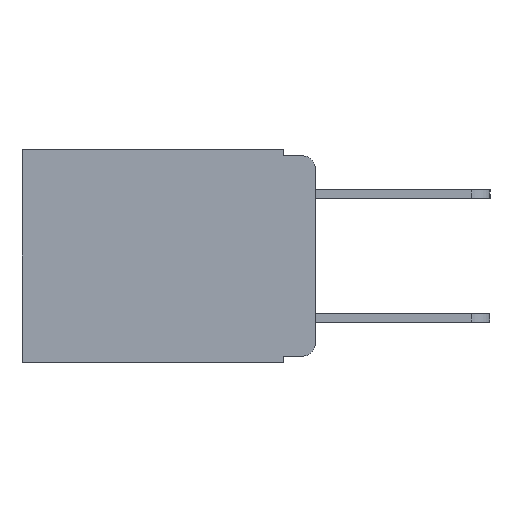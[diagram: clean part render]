
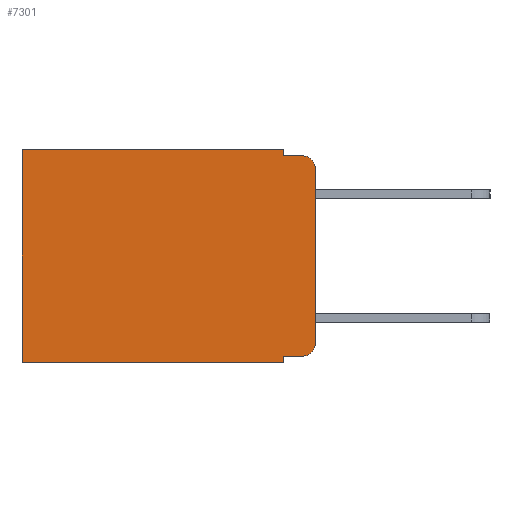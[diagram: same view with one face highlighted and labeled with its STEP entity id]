
A CAD part, left-side view. The second image highlights one B-rep face of the part: STEP entity #7301.
In plain terms, the highlighted planar face has unit normal (-1, 0, 0).
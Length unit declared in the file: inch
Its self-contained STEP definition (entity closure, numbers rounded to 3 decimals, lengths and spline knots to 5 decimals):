
#232 = DIRECTION ( 'NONE',  ( 0., 0., -1. ) ) ;
#924 = LINE ( 'NONE', #11847, #10627 ) ;
#1028 = VECTOR ( 'NONE', #232, 39.37008 ) ;
#1102 = DIRECTION ( 'NONE',  ( 0., 0., -1. ) ) ;
#1113 = DIRECTION ( 'NONE',  ( -1., 0., 0. ) ) ;
#1118 = AXIS2_PLACEMENT_3D ( 'NONE', #11183, #9287, #4000 ) ;
#1119 = CARTESIAN_POINT ( 'NONE',  ( 0.298, 0.02, -0.313 ) ) ;
#1392 = CARTESIAN_POINT ( 'NONE',  ( 0.298, 0.051, -0.343 ) ) ;
#1511 = EDGE_CURVE ( 'NONE', #3085, #6840, #924, .T. ) ;
#1560 = CARTESIAN_POINT ( 'NONE',  ( 0.298, 0.473, 0. ) ) ;
#1775 = EDGE_CURVE ( 'NONE', #11462, #7690, #8368, .T. ) ;
#1790 = PLANE ( 'NONE',  #6377 ) ;
#1794 = VERTEX_POINT ( 'NONE', #3518 ) ;
#1869 = CARTESIAN_POINT ( 'NONE',  ( 0.298, 0.02, -0.01 ) ) ;
#2111 = DIRECTION ( 'NONE',  ( 0., -1., 0. ) ) ;
#2222 = ORIENTED_EDGE ( 'NONE', *, *, #4239, .F. ) ;
#2266 = EDGE_CURVE ( 'NONE', #10200, #12185, #2686, .T. ) ;
#2686 = LINE ( 'NONE', #4710, #9830 ) ;
#2898 = CARTESIAN_POINT ( 'NONE',  ( 0.298, 0.473, 0. ) ) ;
#3085 = VERTEX_POINT ( 'NONE', #1392 ) ;
#3128 = CARTESIAN_POINT ( 'NONE',  ( 0.298, 0., -0.03 ) ) ;
#3170 = EDGE_LOOP ( 'NONE', ( #9669, #8063, #9307, #2222, #4991, #7589, #6895, #10228, #5278, #4367 ) ) ;
#3518 = CARTESIAN_POINT ( 'NONE',  ( 0.298, 0.02, -0.333 ) ) ;
#3519 = CARTESIAN_POINT ( 'NONE',  ( 0.298, 0., -0.313 ) ) ;
#3563 = EDGE_CURVE ( 'NONE', #7358, #12185, #5284, .T. ) ;
#3959 = VECTOR ( 'NONE', #5899, 39.37008 ) ;
#4000 = DIRECTION ( 'NONE',  ( 0., 0., -1. ) ) ;
#4239 = EDGE_CURVE ( 'NONE', #11462, #10200, #5687, .T. ) ;
#4253 = CARTESIAN_POINT ( 'NONE',  ( 0.298, 0., 0. ) ) ;
#4279 = FACE_OUTER_BOUND ( 'NONE', #3170, .T. ) ;
#4367 = ORIENTED_EDGE ( 'NONE', *, *, #7409, .T. ) ;
#4710 = CARTESIAN_POINT ( 'NONE',  ( 0.298, 0.051, -0.01 ) ) ;
#4991 = ORIENTED_EDGE ( 'NONE', *, *, #1775, .T. ) ;
#5025 = CARTESIAN_POINT ( 'NONE',  ( 0.298, 0., 0. ) ) ;
#5060 = CARTESIAN_POINT ( 'NONE',  ( 0.298, 0.051, -0.333 ) ) ;
#5078 = CARTESIAN_POINT ( 'NONE',  ( 0.298, 0.051, 0. ) ) ;
#5278 = ORIENTED_EDGE ( 'NONE', *, *, #6761, .T. ) ;
#5284 = CIRCLE ( 'NONE', #1118, 0.02 ) ;
#5519 = EDGE_CURVE ( 'NONE', #7690, #6840, #11693, .T. ) ;
#5687 = LINE ( 'NONE', #5078, #10234 ) ;
#5846 = VECTOR ( 'NONE', #8536, 39.37008 ) ;
#5899 = DIRECTION ( 'NONE',  ( 0., 0., -1. ) ) ;
#6111 = EDGE_CURVE ( 'NONE', #7524, #3085, #6507, .T. ) ;
#6377 = AXIS2_PLACEMENT_3D ( 'NONE', #4253, #10453, #7131 ) ;
#6491 = CARTESIAN_POINT ( 'NONE',  ( 0.298, 0.051, 0. ) ) ;
#6498 = CARTESIAN_POINT ( 'NONE',  ( 0.298, 0.051, -0.333 ) ) ;
#6507 = LINE ( 'NONE', #12010, #1028 ) ;
#6761 = EDGE_CURVE ( 'NONE', #7524, #1794, #11510, .T. ) ;
#6777 = EDGE_CURVE ( 'NONE', #7358, #11920, #8949, .T. ) ;
#6840 = VERTEX_POINT ( 'NONE', #9971 ) ;
#6895 = ORIENTED_EDGE ( 'NONE', *, *, #1511, .F. ) ;
#6987 = VECTOR ( 'NONE', #7610, 39.37008 ) ;
#7131 = DIRECTION ( 'NONE',  ( 0., 0., -1. ) ) ;
#7301 = ADVANCED_FACE ( 'NONE', ( #4279 ), #1790, .F. ) ;
#7358 = VERTEX_POINT ( 'NONE', #3128 ) ;
#7409 = EDGE_CURVE ( 'NONE', #1794, #11920, #10147, .T. ) ;
#7524 = VERTEX_POINT ( 'NONE', #6498 ) ;
#7589 = ORIENTED_EDGE ( 'NONE', *, *, #5519, .T. ) ;
#7593 = DIRECTION ( 'NONE',  ( 0., 0., -1. ) ) ;
#7610 = DIRECTION ( 'NONE',  ( 0., 0., -1. ) ) ;
#7690 = VERTEX_POINT ( 'NONE', #1560 ) ;
#8063 = ORIENTED_EDGE ( 'NONE', *, *, #3563, .T. ) ;
#8368 = LINE ( 'NONE', #9704, #5846 ) ;
#8536 = DIRECTION ( 'NONE',  ( 0., 1., 0. ) ) ;
#8949 = LINE ( 'NONE', #5025, #3959 ) ;
#9287 = DIRECTION ( 'NONE',  ( -1., 0., 0. ) ) ;
#9307 = ORIENTED_EDGE ( 'NONE', *, *, #2266, .F. ) ;
#9400 = CARTESIAN_POINT ( 'NONE',  ( 0.298, 0.051, -0.01 ) ) ;
#9491 = DIRECTION ( 'NONE',  ( 0., -1., 0. ) ) ;
#9669 = ORIENTED_EDGE ( 'NONE', *, *, #6777, .F. ) ;
#9704 = CARTESIAN_POINT ( 'NONE',  ( 0.298, 0., 0. ) ) ;
#9830 = VECTOR ( 'NONE', #9491, 39.37008 ) ;
#9971 = CARTESIAN_POINT ( 'NONE',  ( 0.298, 0.473, -0.343 ) ) ;
#10147 = CIRCLE ( 'NONE', #10578, 0.02 ) ;
#10200 = VERTEX_POINT ( 'NONE', #9400 ) ;
#10228 = ORIENTED_EDGE ( 'NONE', *, *, #6111, .F. ) ;
#10234 = VECTOR ( 'NONE', #7593, 39.37008 ) ;
#10453 = DIRECTION ( 'NONE',  ( 1., 0., 0. ) ) ;
#10578 = AXIS2_PLACEMENT_3D ( 'NONE', #1119, #1113, #1102 ) ;
#10627 = VECTOR ( 'NONE', #11858, 39.37008 ) ;
#11183 = CARTESIAN_POINT ( 'NONE',  ( 0.298, 0.02, -0.03 ) ) ;
#11230 = VECTOR ( 'NONE', #2111, 39.37008 ) ;
#11462 = VERTEX_POINT ( 'NONE', #6491 ) ;
#11510 = LINE ( 'NONE', #5060, #11230 ) ;
#11693 = LINE ( 'NONE', #2898, #6987 ) ;
#11847 = CARTESIAN_POINT ( 'NONE',  ( 0.298, 0., -0.343 ) ) ;
#11858 = DIRECTION ( 'NONE',  ( 0., 1., 0. ) ) ;
#11920 = VERTEX_POINT ( 'NONE', #3519 ) ;
#12010 = CARTESIAN_POINT ( 'NONE',  ( 0.298, 0.051, 0. ) ) ;
#12185 = VERTEX_POINT ( 'NONE', #1869 ) ;
